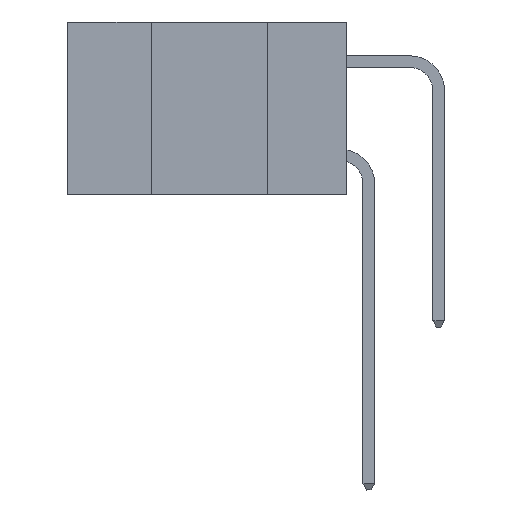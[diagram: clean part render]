
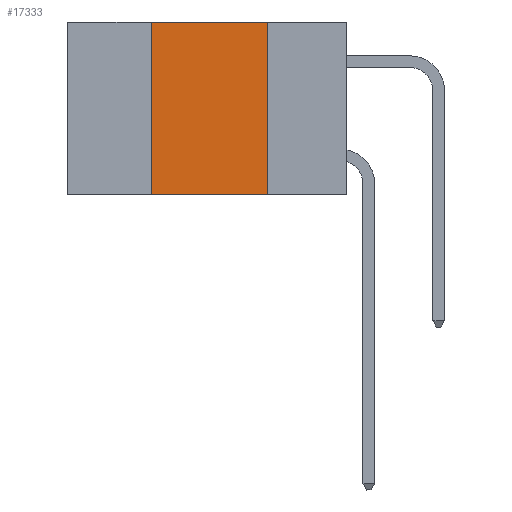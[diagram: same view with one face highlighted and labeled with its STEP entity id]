
A CAD part, left-side view. The second image highlights one B-rep face of the part: STEP entity #17333.
In plain terms, the highlighted planar face has unit normal (-1, 0, 0).
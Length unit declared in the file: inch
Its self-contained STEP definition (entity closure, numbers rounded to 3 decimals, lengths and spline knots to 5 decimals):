
#98 = ORIENTED_EDGE ( 'NONE', *, *, #17597, .T. ) ;
#216 = VERTEX_POINT ( 'NONE', #16067 ) ;
#425 = CARTESIAN_POINT ( 'NONE',  ( 0., 0.6, 0. ) ) ;
#543 = CARTESIAN_POINT ( 'NONE',  ( 0., 0.42, 0. ) ) ;
#634 = DIRECTION ( 'NONE',  ( 0., -1., 0. ) ) ;
#655 = VERTEX_POINT ( 'NONE', #8898 ) ;
#1697 = VECTOR ( 'NONE', #14698, 39.37008 ) ;
#4700 = PLANE ( 'NONE',  #20948 ) ;
#4868 = EDGE_CURVE ( 'NONE', #216, #655, #17871, .T. ) ;
#5216 = EDGE_CURVE ( 'NONE', #13789, #216, #15304, .T. ) ;
#6150 = EDGE_LOOP ( 'NONE', ( #12855, #17862, #15700, #98 ) ) ;
#6332 = DIRECTION ( 'NONE',  ( 0., 0., -1. ) ) ;
#6555 = LINE ( 'NONE', #19486, #1697 ) ;
#8572 = DIRECTION ( 'NONE',  ( 0., 0., -1. ) ) ;
#8898 = CARTESIAN_POINT ( 'NONE',  ( 0., 0.17, -0.37 ) ) ;
#9510 = CARTESIAN_POINT ( 'NONE',  ( 0., 0.17, 0. ) ) ;
#10966 = VECTOR ( 'NONE', #634, 39.37008 ) ;
#11012 = FACE_OUTER_BOUND ( 'NONE', #6150, .T. ) ;
#11126 = LINE ( 'NONE', #14424, #13159 ) ;
#11304 = CARTESIAN_POINT ( 'NONE',  ( 0., 0.6, 0. ) ) ;
#12855 = ORIENTED_EDGE ( 'NONE', *, *, #4868, .F. ) ;
#13159 = VECTOR ( 'NONE', #14635, 39.37008 ) ;
#13289 = VERTEX_POINT ( 'NONE', #14355 ) ;
#13789 = VERTEX_POINT ( 'NONE', #543 ) ;
#14269 = EDGE_CURVE ( 'NONE', #13289, #13789, #11126, .T. ) ;
#14355 = CARTESIAN_POINT ( 'NONE',  ( 0., 0.42, -0.37 ) ) ;
#14424 = CARTESIAN_POINT ( 'NONE',  ( 0., 0.42, 0. ) ) ;
#14635 = DIRECTION ( 'NONE',  ( 0., 0., 1. ) ) ;
#14698 = DIRECTION ( 'NONE',  ( 0., -1., 0. ) ) ;
#15304 = LINE ( 'NONE', #425, #10966 ) ;
#15557 = VECTOR ( 'NONE', #8572, 39.37008 ) ;
#15700 = ORIENTED_EDGE ( 'NONE', *, *, #14269, .F. ) ;
#16067 = CARTESIAN_POINT ( 'NONE',  ( 0., 0.17, 0. ) ) ;
#16072 = DIRECTION ( 'NONE',  ( 1., 0., 0. ) ) ;
#17333 = ADVANCED_FACE ( 'NONE', ( #11012 ), #4700, .F. ) ;
#17597 = EDGE_CURVE ( 'NONE', #13289, #655, #6555, .T. ) ;
#17862 = ORIENTED_EDGE ( 'NONE', *, *, #5216, .F. ) ;
#17871 = LINE ( 'NONE', #9510, #15557 ) ;
#19486 = CARTESIAN_POINT ( 'NONE',  ( 0., 0.6, -0.37 ) ) ;
#20948 = AXIS2_PLACEMENT_3D ( 'NONE', #11304, #16072, #6332 ) ;
